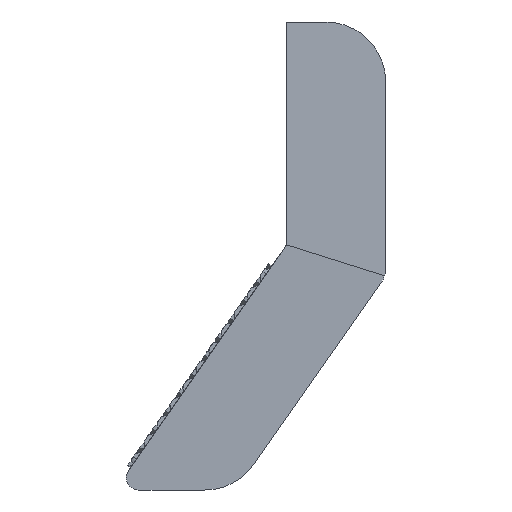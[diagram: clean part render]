
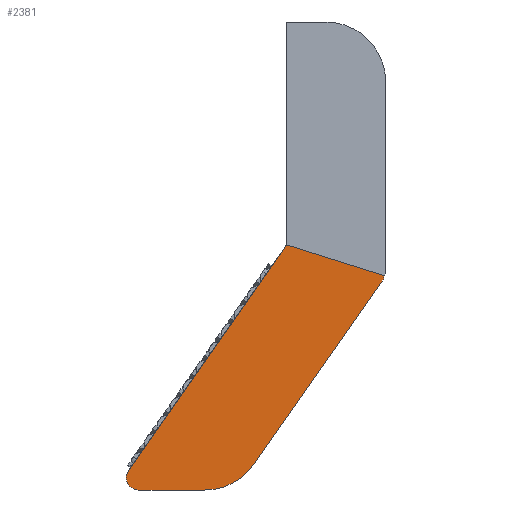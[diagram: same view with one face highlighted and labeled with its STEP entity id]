
A CAD part, left-side view. The second image highlights one B-rep face of the part: STEP entity #2381.
In plain terms, the highlighted planar face has unit normal (-0.999, -0.033, -0.023).
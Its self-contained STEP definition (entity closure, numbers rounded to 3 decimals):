
#493 = EDGE_LOOP ( 'NONE', ( #7536, #3865, #18155, #6717, #15593, #14323, #11206, #4461 ) ) ;
#1670 = CARTESIAN_POINT ( 'NONE',  ( -8.89, 5.259, -70.614 ) ) ;
#1941 = VECTOR ( 'NONE', #3827, 1000. ) ;
#2122 = PLANE ( 'NONE',  #7511 ) ;
#2316 =( BOUNDED_CURVE ( )  B_SPLINE_CURVE ( 3, ( #12573, #5455, #13985, #5511 ),
 .UNSPECIFIED., .F., .T. ) 
 B_SPLINE_CURVE_WITH_KNOTS ( ( 4, 4 ),
 ( 0.96, 3.142 ),
 .UNSPECIFIED. ) 
 CURVE ( )  GEOMETRIC_REPRESENTATION_ITEM ( )  RATIONAL_B_SPLINE_CURVE ( ( 1., 0.641, 0.641, 1. ) ) 
 REPRESENTATION_ITEM ( '' )  );
#2381 = ADVANCED_FACE ( 'NONE', ( #9212 ), #2122, .F. ) ;
#3568 = DIRECTION ( 'NONE',  ( -0.033, 0.999, 0. ) ) ;
#3791 = VERTEX_POINT ( 'NONE', #5245 ) ;
#3827 = DIRECTION ( 'NONE',  ( 0., 0.574, -0.819 ) ) ;
#3865 = ORIENTED_EDGE ( 'NONE', *, *, #7303, .F. ) ;
#3929 = EDGE_CURVE ( 'NONE', #3791, #15557, #13925, .T. ) ;
#4245 = CARTESIAN_POINT ( 'NONE',  ( -9.525, 0.061, -35.626 ) ) ;
#4461 = ORIENTED_EDGE ( 'NONE', *, *, #11545, .F. ) ;
#4647 = CARTESIAN_POINT ( 'NONE',  ( -8.896, -15.652, -40.495 ) ) ;
#4942 = CARTESIAN_POINT ( 'NONE',  ( -8.634, -22.173, -42.551 ) ) ;
#5245 = CARTESIAN_POINT ( 'NONE',  ( -9.525, 0.144, -35.765 ) ) ;
#5286 =( BOUNDED_CURVE ( )  B_SPLINE_CURVE ( 3, ( #14464, #15875, #7416, #17328 ),
 .UNSPECIFIED., .F., .T. ) 
 B_SPLINE_CURVE_WITH_KNOTS ( ( 4, 4 ),
 ( 0., 0.96 ),
 .UNSPECIFIED. ) 
 CURVE ( )  GEOMETRIC_REPRESENTATION_ITEM ( )  RATIONAL_B_SPLINE_CURVE ( ( 1., 0.925, 0.925, 1. ) ) 
 REPRESENTATION_ITEM ( '' )  );
#5417 = VERTEX_POINT ( 'NONE', #11227 ) ;
#5455 = CARTESIAN_POINT ( 'NONE',  ( -9.46, 25.408, -74.676 ) ) ;
#5511 = CARTESIAN_POINT ( 'NONE',  ( -9.525, 25.203, -71.553 ) ) ;
#5642 = EDGE_CURVE ( 'NONE', #18008, #14652, #17572, .T. ) ;
#5722 = VERTEX_POINT ( 'NONE', #16237 ) ;
#6108 = CARTESIAN_POINT ( 'NONE',  ( -8.89, -15.225, -41.361 ) ) ;
#6362 = VECTOR ( 'NONE', #11539, 1000. ) ;
#6717 = ORIENTED_EDGE ( 'NONE', *, *, #15186, .T. ) ;
#6955 = CARTESIAN_POINT ( 'NONE',  ( -8.89, -15.225, -41.361 ) ) ;
#6982 = CARTESIAN_POINT ( 'NONE',  ( -9.525, 0.144, -35.765 ) ) ;
#7201 = VERTEX_POINT ( 'NONE', #1670 ) ;
#7303 = EDGE_CURVE ( 'NONE', #15557, #18008, #15549, .T. ) ;
#7416 = CARTESIAN_POINT ( 'NONE',  ( -8.949, 9.89, -74.676 ) ) ;
#7445 = CARTESIAN_POINT ( 'NONE',  ( -8.892, -15.554, -40.805 ) ) ;
#7511 = AXIS2_PLACEMENT_3D ( 'NONE', #4942, #12063, #3568 ) ;
#7536 = ORIENTED_EDGE ( 'NONE', *, *, #5642, .F. ) ;
#7583 = VECTOR ( 'NONE', #13211, 1000. ) ;
#8249 = CARTESIAN_POINT ( 'NONE',  ( -9.525, 25.203, -71.553 ) ) ;
#8704 = CARTESIAN_POINT ( 'NONE',  ( -9.399, 23.577, -74.676 ) ) ;
#9212 = FACE_OUTER_BOUND ( 'NONE', #493, .T. ) ;
#10705 = CARTESIAN_POINT ( 'NONE',  ( -9.525, 25.203, -71.553 ) ) ;
#11206 = ORIENTED_EDGE ( 'NONE', *, *, #13778, .F. ) ;
#11227 = CARTESIAN_POINT ( 'NONE',  ( -9.053, 13.061, -74.676 ) ) ;
#11539 = DIRECTION ( 'NONE',  ( 0.033, -0.999, 0. ) ) ;
#11545 = EDGE_CURVE ( 'NONE', #14652, #7201, #17033, .T. ) ;
#11671 = CARTESIAN_POINT ( 'NONE',  ( -8.89, -15.411, -41.096 ) ) ;
#11828 = CARTESIAN_POINT ( 'NONE',  ( -9.526, 0.037, -35.548 ) ) ;
#12063 = DIRECTION ( 'NONE',  ( 0.999, 0.033, 0.023 ) ) ;
#12573 = CARTESIAN_POINT ( 'NONE',  ( -9.399, 23.577, -74.676 ) ) ;
#12814 = VECTOR ( 'NONE', #18129, 1000. ) ;
#13211 = DIRECTION ( 'NONE',  ( 0.038, -0.953, -0.3 ) ) ;
#13252 = LINE ( 'NONE', #8249, #12814 ) ;
#13719 = CARTESIAN_POINT ( 'NONE',  ( -8.89, -15.225, -41.361 ) ) ;
#13778 = EDGE_CURVE ( 'NONE', #7201, #5417, #5286, .T. ) ;
#13925 =( BOUNDED_CURVE ( )  B_SPLINE_CURVE ( 3, ( #6982, #16950, #4245, #14135 ),
 .UNSPECIFIED., .F., .T. ) 
 B_SPLINE_CURVE_WITH_KNOTS ( ( 4, 4 ),
 ( 3.142, 3.447 ),
 .UNSPECIFIED. ) 
 CURVE ( )  GEOMETRIC_REPRESENTATION_ITEM ( )  RATIONAL_B_SPLINE_CURVE ( ( 1., 0.992, 0.992, 1. ) ) 
 REPRESENTATION_ITEM ( '' )  );
#13985 = CARTESIAN_POINT ( 'NONE',  ( -9.525, 26.253, -73.053 ) ) ;
#14009 = VERTEX_POINT ( 'NONE', #10705 ) ;
#14135 = CARTESIAN_POINT ( 'NONE',  ( -9.526, 0.037, -35.548 ) ) ;
#14323 = ORIENTED_EDGE ( 'NONE', *, *, #16152, .T. ) ;
#14464 = CARTESIAN_POINT ( 'NONE',  ( -8.89, 5.259, -70.614 ) ) ;
#14652 = VERTEX_POINT ( 'NONE', #6955 ) ;
#15186 = EDGE_CURVE ( 'NONE', #3791, #14009, #13252, .T. ) ;
#15549 = LINE ( 'NONE', #15997, #7583 ) ;
#15557 = VERTEX_POINT ( 'NONE', #11828 ) ;
#15593 = ORIENTED_EDGE ( 'NONE', *, *, #16605, .F. ) ;
#15875 = CARTESIAN_POINT ( 'NONE',  ( -8.89, 7.077, -73.212 ) ) ;
#15908 = CARTESIAN_POINT ( 'NONE',  ( -8.896, -15.652, -40.495 ) ) ;
#15997 = CARTESIAN_POINT ( 'NONE',  ( -9.526, 0.037, -35.548 ) ) ;
#16152 = EDGE_CURVE ( 'NONE', #5722, #5417, #17644, .T. ) ;
#16237 = CARTESIAN_POINT ( 'NONE',  ( -9.399, 23.577, -74.676 ) ) ;
#16605 = EDGE_CURVE ( 'NONE', #5722, #14009, #2316, .T. ) ;
#16950 = CARTESIAN_POINT ( 'NONE',  ( -9.525, 0.097, -35.699 ) ) ;
#17033 = LINE ( 'NONE', #13719, #1941 ) ;
#17328 = CARTESIAN_POINT ( 'NONE',  ( -9.053, 13.061, -74.676 ) ) ;
#17572 =( BOUNDED_CURVE ( )  B_SPLINE_CURVE ( 3, ( #4647, #7445, #11671, #6108 ),
 .UNSPECIFIED., .F., .T. ) 
 B_SPLINE_CURVE_WITH_KNOTS ( ( 4, 4 ),
 ( 5.978, 6.283 ),
 .UNSPECIFIED. ) 
 CURVE ( )  GEOMETRIC_REPRESENTATION_ITEM ( )  RATIONAL_B_SPLINE_CURVE ( ( 1., 0.992, 0.992, 1. ) ) 
 REPRESENTATION_ITEM ( '' )  );
#17644 = LINE ( 'NONE', #8704, #6362 ) ;
#18008 = VERTEX_POINT ( 'NONE', #15908 ) ;
#18129 = DIRECTION ( 'NONE',  ( 0., 0.574, -0.819 ) ) ;
#18155 = ORIENTED_EDGE ( 'NONE', *, *, #3929, .F. ) ;
